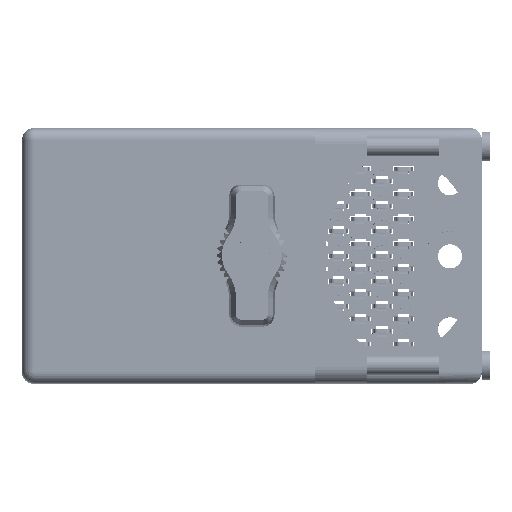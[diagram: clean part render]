
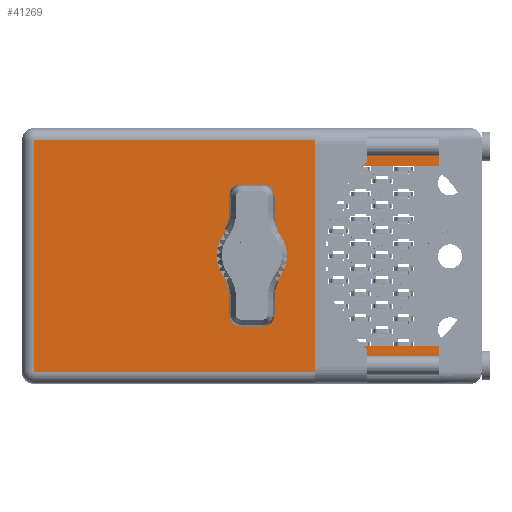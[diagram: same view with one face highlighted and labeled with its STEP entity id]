
A CAD part, top view. The second image highlights one B-rep face of the part: STEP entity #41269.
In plain terms, the highlighted face is planar.
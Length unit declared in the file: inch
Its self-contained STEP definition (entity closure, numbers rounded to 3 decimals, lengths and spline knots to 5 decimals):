
#3384 = VECTOR ( 'NONE', #40068, 39.37008 ) ;
#4056 = DIRECTION ( 'NONE',  ( 0., 0., -1. ) ) ;
#5576 = ORIENTED_EDGE ( 'NONE', *, *, #6894, .F. ) ;
#5632 = CARTESIAN_POINT ( 'NONE',  ( -1.3775, 1.93, -0.695 ) ) ;
#6893 = CARTESIAN_POINT ( 'NONE',  ( 1.1215, 1.93, 0.54 ) ) ;
#6894 = EDGE_CURVE ( 'NONE', #98166, #12654, #31630, .T. ) ;
#7180 = CARTESIAN_POINT ( 'NONE',  ( 1.1215, 1.93, -0.765 ) ) ;
#9538 = ORIENTED_EDGE ( 'NONE', *, *, #38825, .F. ) ;
#10039 = CARTESIAN_POINT ( 'NONE',  ( 0., 1.93, 0. ) ) ;
#10405 = FACE_OUTER_BOUND ( 'NONE', #41387, .T. ) ;
#10410 = DIRECTION ( 'NONE',  ( 0., 0., 1. ) ) ;
#12319 = VERTEX_POINT ( 'NONE', #94326 ) ;
#12654 = VERTEX_POINT ( 'NONE', #28742 ) ;
#12848 = VERTEX_POINT ( 'NONE', #50174 ) ;
#13089 = LINE ( 'NONE', #20179, #75701 ) ;
#17422 = CARTESIAN_POINT ( 'NONE',  ( 0.4075, 1.93, -0.54 ) ) ;
#19835 = CARTESIAN_POINT ( 'NONE',  ( 0.4075, 1.93, 0.54 ) ) ;
#20179 = CARTESIAN_POINT ( 'NONE',  ( 0.4075, 1.93, -0.54 ) ) ;
#22471 = DIRECTION ( 'NONE',  ( -1., 0., 0. ) ) ;
#24025 = DIRECTION ( 'NONE',  ( 0., 1., 0. ) ) ;
#25119 = CARTESIAN_POINT ( 'NONE',  ( 1.1215, 1.93, -0.765 ) ) ;
#25167 = CARTESIAN_POINT ( 'NONE',  ( 1.1215, 1.93, 0.54 ) ) ;
#28742 = CARTESIAN_POINT ( 'NONE',  ( 1.1215, 1.93, 0.695 ) ) ;
#31630 = LINE ( 'NONE', #7180, #3384 ) ;
#32515 = VERTEX_POINT ( 'NONE', #70038 ) ;
#32827 = DIRECTION ( 'NONE',  ( 1., 0., 0. ) ) ;
#34235 = EDGE_CURVE ( 'NONE', #12848, #70062, #56358, .T. ) ;
#35262 = DIRECTION ( 'NONE',  ( -1., 0., 0. ) ) ;
#35619 = DIRECTION ( 'NONE',  ( 0., 1., 0. ) ) ;
#36048 = AXIS2_PLACEMENT_3D ( 'NONE', #68137, #35619, #35262 ) ;
#36334 = EDGE_CURVE ( 'NONE', #70062, #12848, #61101, .T. ) ;
#38388 = VECTOR ( 'NONE', #32827, 39.37008 ) ;
#38825 = EDGE_CURVE ( 'NONE', #53721, #32515, #87331, .T. ) ;
#38978 = DIRECTION ( 'NONE',  ( 0., 1., 0. ) ) ;
#39076 = DIRECTION ( 'NONE',  ( -1., 0., 0. ) ) ;
#40068 = DIRECTION ( 'NONE',  ( 0., 0., 1. ) ) ;
#41269 = ADVANCED_FACE ( 'NONE', ( #10405, #94783 ), #60614, .T. ) ;
#41387 = EDGE_LOOP ( 'NONE', ( #48774, #79761, #5576, #44059, #66498, #77689, #9538, #98633 ) ) ;
#44059 = ORIENTED_EDGE ( 'NONE', *, *, #101061, .T. ) ;
#44600 = ORIENTED_EDGE ( 'NONE', *, *, #36334, .F. ) ;
#45137 = AXIS2_PLACEMENT_3D ( 'NONE', #80061, #38978, #62602 ) ;
#48774 = ORIENTED_EDGE ( 'NONE', *, *, #79036, .T. ) ;
#50076 = EDGE_CURVE ( 'NONE', #57929, #57729, #13089, .T. ) ;
#50174 = CARTESIAN_POINT ( 'NONE',  ( 0., 1.93, -0.17 ) ) ;
#53721 = VERTEX_POINT ( 'NONE', #93047 ) ;
#56358 = CIRCLE ( 'NONE', #68958, 0.17 ) ;
#57380 = ORIENTED_EDGE ( 'NONE', *, *, #34235, .F. ) ;
#57729 = VERTEX_POINT ( 'NONE', #17422 ) ;
#57929 = VERTEX_POINT ( 'NONE', #19835 ) ;
#58248 = CARTESIAN_POINT ( 'NONE',  ( -1.3075, 1.93, -0.765 ) ) ;
#59657 = CARTESIAN_POINT ( 'NONE',  ( -1.3075, 1.93, -0.695 ) ) ;
#60614 = PLANE ( 'NONE',  #36048 ) ;
#61101 = CIRCLE ( 'NONE', #45137, 0.17 ) ;
#62602 = DIRECTION ( 'NONE',  ( 0., 0., 1. ) ) ;
#63141 = LINE ( 'NONE', #5632, #73363 ) ;
#64427 = VECTOR ( 'NONE', #10410, 39.37008 ) ;
#66498 = ORIENTED_EDGE ( 'NONE', *, *, #50076, .T. ) ;
#66620 = CARTESIAN_POINT ( 'NONE',  ( 1.1215, 1.93, -0.54 ) ) ;
#66747 = EDGE_CURVE ( 'NONE', #12319, #12654, #84423, .T. ) ;
#68137 = CARTESIAN_POINT ( 'NONE',  ( -1.3775, 1.93, -0.765 ) ) ;
#68958 = AXIS2_PLACEMENT_3D ( 'NONE', #10039, #24025, #97231 ) ;
#70038 = CARTESIAN_POINT ( 'NONE',  ( 1.1215, 1.93, -0.54 ) ) ;
#70062 = VERTEX_POINT ( 'NONE', #97692 ) ;
#70099 = EDGE_CURVE ( 'NONE', #57729, #32515, #100241, .T. ) ;
#72350 = LINE ( 'NONE', #6893, #82567 ) ;
#73151 = LINE ( 'NONE', #58248, #92272 ) ;
#73363 = VECTOR ( 'NONE', #22471, 39.37008 ) ;
#75701 = VECTOR ( 'NONE', #4056, 39.37008 ) ;
#75865 = DIRECTION ( 'NONE',  ( 1., 0., 0. ) ) ;
#77689 = ORIENTED_EDGE ( 'NONE', *, *, #70099, .T. ) ;
#79036 = EDGE_CURVE ( 'NONE', #103669, #12319, #73151, .T. ) ;
#79761 = ORIENTED_EDGE ( 'NONE', *, *, #66747, .T. ) ;
#79800 = VECTOR ( 'NONE', #75865, 39.37008 ) ;
#80061 = CARTESIAN_POINT ( 'NONE',  ( 0., 1.93, 0. ) ) ;
#81708 = CARTESIAN_POINT ( 'NONE',  ( 1.1215, 1.93, 0.695 ) ) ;
#82567 = VECTOR ( 'NONE', #39076, 39.37008 ) ;
#84423 = LINE ( 'NONE', #81708, #38388 ) ;
#87266 = EDGE_LOOP ( 'NONE', ( #44600, #57380 ) ) ;
#87331 = LINE ( 'NONE', #25119, #64427 ) ;
#92272 = VECTOR ( 'NONE', #92874, 39.37008 ) ;
#92874 = DIRECTION ( 'NONE',  ( 0., 0., 1. ) ) ;
#93047 = CARTESIAN_POINT ( 'NONE',  ( 1.1215, 1.93, -0.695 ) ) ;
#94326 = CARTESIAN_POINT ( 'NONE',  ( -1.3075, 1.93, 0.695 ) ) ;
#94783 = FACE_BOUND ( 'NONE', #87266, .T. ) ;
#97231 = DIRECTION ( 'NONE',  ( 0., 0., 1. ) ) ;
#97692 = CARTESIAN_POINT ( 'NONE',  ( 0., 1.93, 0.17 ) ) ;
#98166 = VERTEX_POINT ( 'NONE', #25167 ) ;
#98633 = ORIENTED_EDGE ( 'NONE', *, *, #102304, .T. ) ;
#100241 = LINE ( 'NONE', #66620, #79800 ) ;
#101061 = EDGE_CURVE ( 'NONE', #98166, #57929, #72350, .T. ) ;
#102304 = EDGE_CURVE ( 'NONE', #53721, #103669, #63141, .T. ) ;
#103669 = VERTEX_POINT ( 'NONE', #59657 ) ;
